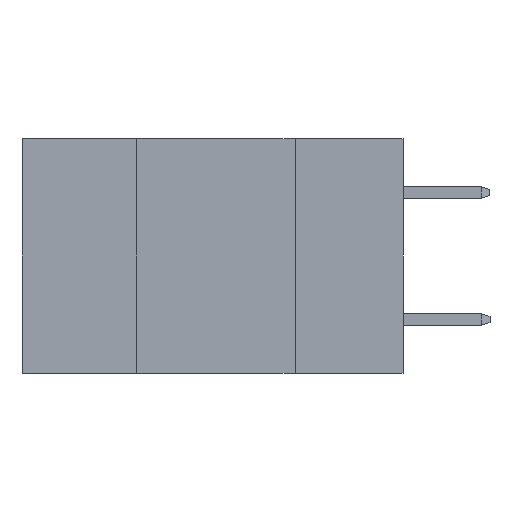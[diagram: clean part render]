
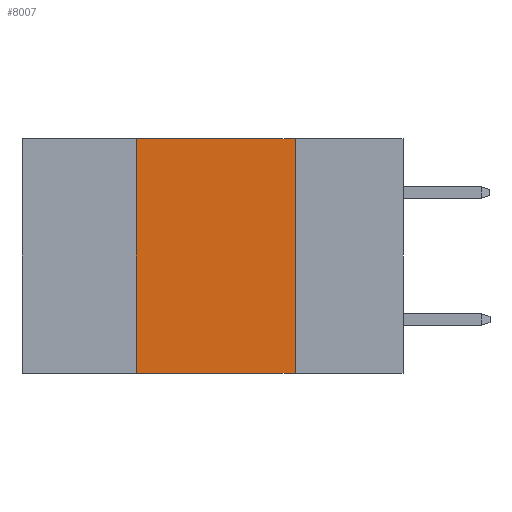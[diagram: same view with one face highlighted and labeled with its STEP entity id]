
A CAD part, left-side view. The second image highlights one B-rep face of the part: STEP entity #8007.
In plain terms, the highlighted planar face has unit normal (-1, 0, 0).
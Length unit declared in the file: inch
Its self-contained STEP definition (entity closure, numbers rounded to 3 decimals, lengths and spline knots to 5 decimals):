
#55 = CARTESIAN_POINT ( 'NONE',  ( 0., 0.42, -0.37 ) ) ;
#723 = DIRECTION ( 'NONE',  ( 0., -1., 0. ) ) ;
#807 = VERTEX_POINT ( 'NONE', #999 ) ;
#999 = CARTESIAN_POINT ( 'NONE',  ( 0., 0.42, 0. ) ) ;
#1639 = EDGE_CURVE ( 'NONE', #6385, #807, #2831, .T. ) ;
#2509 = CARTESIAN_POINT ( 'NONE',  ( 0., 0.17, -0.37 ) ) ;
#2831 = LINE ( 'NONE', #4249, #3184 ) ;
#2985 = LINE ( 'NONE', #9730, #4155 ) ;
#3184 = VECTOR ( 'NONE', #9668, 39.37008 ) ;
#3395 = ORIENTED_EDGE ( 'NONE', *, *, #1639, .F. ) ;
#4155 = VECTOR ( 'NONE', #723, 39.37008 ) ;
#4249 = CARTESIAN_POINT ( 'NONE',  ( 0., 0.42, 0. ) ) ;
#4353 = EDGE_CURVE ( 'NONE', #807, #8538, #2985, .T. ) ;
#4606 = ORIENTED_EDGE ( 'NONE', *, *, #4353, .F. ) ;
#4654 = EDGE_CURVE ( 'NONE', #6385, #4978, #6835, .T. ) ;
#4712 = EDGE_CURVE ( 'NONE', #8538, #4978, #5179, .T. ) ;
#4794 = CARTESIAN_POINT ( 'NONE',  ( 0., 0.6, 0. ) ) ;
#4978 = VERTEX_POINT ( 'NONE', #2509 ) ;
#5021 = CARTESIAN_POINT ( 'NONE',  ( 0., 0.17, 0. ) ) ;
#5143 = ORIENTED_EDGE ( 'NONE', *, *, #4654, .T. ) ;
#5179 = LINE ( 'NONE', #7398, #6035 ) ;
#5562 = VECTOR ( 'NONE', #8964, 39.37008 ) ;
#5724 = FACE_OUTER_BOUND ( 'NONE', #8481, .T. ) ;
#5751 = AXIS2_PLACEMENT_3D ( 'NONE', #4794, #7804, #9726 ) ;
#5798 = ORIENTED_EDGE ( 'NONE', *, *, #4712, .F. ) ;
#5999 = CARTESIAN_POINT ( 'NONE',  ( 0., 0.6, -0.37 ) ) ;
#6035 = VECTOR ( 'NONE', #8156, 39.37008 ) ;
#6385 = VERTEX_POINT ( 'NONE', #55 ) ;
#6835 = LINE ( 'NONE', #5999, #5562 ) ;
#7398 = CARTESIAN_POINT ( 'NONE',  ( 0., 0.17, 0. ) ) ;
#7804 = DIRECTION ( 'NONE',  ( 1., 0., 0. ) ) ;
#8007 = ADVANCED_FACE ( 'NONE', ( #5724 ), #8774, .F. ) ;
#8156 = DIRECTION ( 'NONE',  ( 0., 0., -1. ) ) ;
#8481 = EDGE_LOOP ( 'NONE', ( #5798, #4606, #3395, #5143 ) ) ;
#8538 = VERTEX_POINT ( 'NONE', #5021 ) ;
#8774 = PLANE ( 'NONE',  #5751 ) ;
#8964 = DIRECTION ( 'NONE',  ( 0., -1., 0. ) ) ;
#9668 = DIRECTION ( 'NONE',  ( 0., 0., 1. ) ) ;
#9726 = DIRECTION ( 'NONE',  ( 0., 0., -1. ) ) ;
#9730 = CARTESIAN_POINT ( 'NONE',  ( 0., 0.6, 0. ) ) ;
